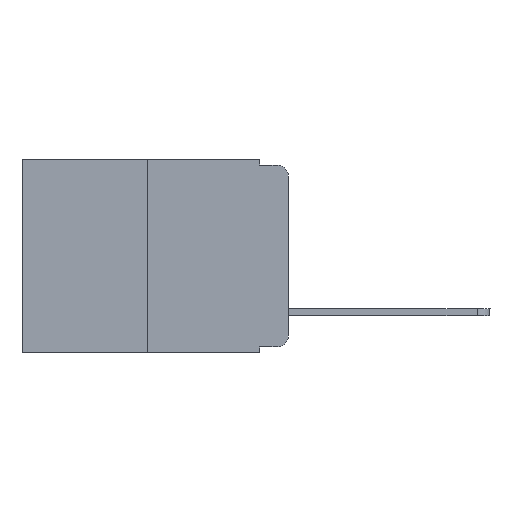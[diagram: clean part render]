
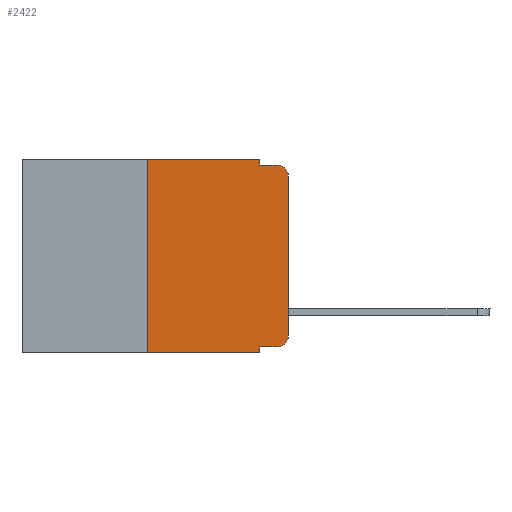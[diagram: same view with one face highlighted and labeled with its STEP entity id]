
A CAD part, left-side view. The second image highlights one B-rep face of the part: STEP entity #2422.
In plain terms, the highlighted planar face has unit normal (-1, 0, 0).
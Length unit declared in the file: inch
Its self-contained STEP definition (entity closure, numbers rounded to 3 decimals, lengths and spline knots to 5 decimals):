
#66 = CARTESIAN_POINT ( 'NONE',  ( 0., 0.25, 0. ) ) ;
#70 = CARTESIAN_POINT ( 'NONE',  ( 0., 0.051, -0.333 ) ) ;
#91 = CARTESIAN_POINT ( 'NONE',  ( 0., 0., -0.313 ) ) ;
#331 = ORIENTED_EDGE ( 'NONE', *, *, #2631, .T. ) ;
#383 = CARTESIAN_POINT ( 'NONE',  ( 0., 0.051, 0. ) ) ;
#431 = CARTESIAN_POINT ( 'NONE',  ( 0., 0.051, -0.343 ) ) ;
#577 = DIRECTION ( 'NONE',  ( 0., 0., -1. ) ) ;
#606 = EDGE_CURVE ( 'NONE', #12456, #6065, #13124, .T. ) ;
#678 = ORIENTED_EDGE ( 'NONE', *, *, #8364, .F. ) ;
#809 = PLANE ( 'NONE',  #10566 ) ;
#844 = CARTESIAN_POINT ( 'NONE',  ( 0., 0.051, -0.01 ) ) ;
#884 = CARTESIAN_POINT ( 'NONE',  ( 0., 0.02, -0.01 ) ) ;
#1283 = CARTESIAN_POINT ( 'NONE',  ( 0., 0., 0. ) ) ;
#1516 = LINE ( 'NONE', #11764, #2070 ) ;
#1545 = DIRECTION ( 'NONE',  ( 0., 0., 1. ) ) ;
#1553 = CARTESIAN_POINT ( 'NONE',  ( 0., 0.051, -0.01 ) ) ;
#1584 = EDGE_CURVE ( 'NONE', #11818, #4936, #2706, .T. ) ;
#1667 = DIRECTION ( 'NONE',  ( 0., 0., -1. ) ) ;
#1796 = DIRECTION ( 'NONE',  ( 1., 0., 0. ) ) ;
#1848 = CIRCLE ( 'NONE', #9337, 0.02 ) ;
#2070 = VECTOR ( 'NONE', #577, 39.37008 ) ;
#2153 = LINE ( 'NONE', #12272, #10392 ) ;
#2422 = ADVANCED_FACE ( 'NONE', ( #10788 ), #809, .F. ) ;
#2631 = EDGE_CURVE ( 'NONE', #3599, #6007, #12322, .T. ) ;
#2706 = LINE ( 'NONE', #844, #4121 ) ;
#3123 = VERTEX_POINT ( 'NONE', #431 ) ;
#3368 = ORIENTED_EDGE ( 'NONE', *, *, #606, .F. ) ;
#3408 = DIRECTION ( 'NONE',  ( 0., 0., -1. ) ) ;
#3510 = VERTEX_POINT ( 'NONE', #91 ) ;
#3599 = VERTEX_POINT ( 'NONE', #6467 ) ;
#3924 = EDGE_CURVE ( 'NONE', #3599, #3123, #12708, .T. ) ;
#4121 = VECTOR ( 'NONE', #10142, 39.37008 ) ;
#4555 = DIRECTION ( 'NONE',  ( 0., 0., -1. ) ) ;
#4722 = ORIENTED_EDGE ( 'NONE', *, *, #5256, .T. ) ;
#4901 = CARTESIAN_POINT ( 'NONE',  ( 0., 0.473, 0. ) ) ;
#4936 = VERTEX_POINT ( 'NONE', #884 ) ;
#5237 = DIRECTION ( 'NONE',  ( 0., -1., 0. ) ) ;
#5256 = EDGE_CURVE ( 'NONE', #6007, #3510, #1848, .T. ) ;
#5392 = EDGE_LOOP ( 'NONE', ( #12470, #13160, #11959, #7307, #3368, #678, #12584, #7066, #331, #4722 ) ) ;
#5424 = CARTESIAN_POINT ( 'NONE',  ( 0., 0.051, 0. ) ) ;
#5482 = VERTEX_POINT ( 'NONE', #6631 ) ;
#5528 = EDGE_CURVE ( 'NONE', #6065, #11818, #1516, .T. ) ;
#5584 = CARTESIAN_POINT ( 'NONE',  ( 0., 0.25, 0. ) ) ;
#5671 = EDGE_CURVE ( 'NONE', #3510, #5482, #6401, .T. ) ;
#5672 = EDGE_CURVE ( 'NONE', #8220, #3123, #2153, .T. ) ;
#6007 = VERTEX_POINT ( 'NONE', #6176 ) ;
#6065 = VERTEX_POINT ( 'NONE', #383 ) ;
#6118 = DIRECTION ( 'NONE',  ( 0., -1., 0. ) ) ;
#6159 = AXIS2_PLACEMENT_3D ( 'NONE', #7482, #10285, #12546 ) ;
#6176 = CARTESIAN_POINT ( 'NONE',  ( 0., 0.02, -0.333 ) ) ;
#6401 = LINE ( 'NONE', #1283, #6568 ) ;
#6467 = CARTESIAN_POINT ( 'NONE',  ( 0., 0.051, -0.333 ) ) ;
#6538 = EDGE_CURVE ( 'NONE', #5482, #4936, #7645, .T. ) ;
#6568 = VECTOR ( 'NONE', #10196, 39.37008 ) ;
#6631 = CARTESIAN_POINT ( 'NONE',  ( 0., 0., -0.03 ) ) ;
#6787 = LINE ( 'NONE', #5584, #8789 ) ;
#7066 = ORIENTED_EDGE ( 'NONE', *, *, #3924, .F. ) ;
#7307 = ORIENTED_EDGE ( 'NONE', *, *, #5528, .F. ) ;
#7482 = CARTESIAN_POINT ( 'NONE',  ( 0., 0.02, -0.03 ) ) ;
#7645 = CIRCLE ( 'NONE', #6159, 0.02 ) ;
#8220 = VERTEX_POINT ( 'NONE', #10468 ) ;
#8364 = EDGE_CURVE ( 'NONE', #8220, #12456, #6787, .T. ) ;
#8789 = VECTOR ( 'NONE', #1545, 39.37008 ) ;
#9337 = AXIS2_PLACEMENT_3D ( 'NONE', #10518, #12585, #3408 ) ;
#9461 = VECTOR ( 'NONE', #11072, 39.37008 ) ;
#10142 = DIRECTION ( 'NONE',  ( 0., -1., 0. ) ) ;
#10196 = DIRECTION ( 'NONE',  ( 0., 0., 1. ) ) ;
#10285 = DIRECTION ( 'NONE',  ( -1., 0., 0. ) ) ;
#10392 = VECTOR ( 'NONE', #5237, 39.37008 ) ;
#10468 = CARTESIAN_POINT ( 'NONE',  ( 0., 0.25, -0.343 ) ) ;
#10518 = CARTESIAN_POINT ( 'NONE',  ( 0., 0.02, -0.313 ) ) ;
#10566 = AXIS2_PLACEMENT_3D ( 'NONE', #11995, #1796, #1667 ) ;
#10787 = VECTOR ( 'NONE', #6118, 39.37008 ) ;
#10788 = FACE_OUTER_BOUND ( 'NONE', #5392, .T. ) ;
#11072 = DIRECTION ( 'NONE',  ( 0., -1., 0. ) ) ;
#11764 = CARTESIAN_POINT ( 'NONE',  ( 0., 0.051, 0. ) ) ;
#11818 = VERTEX_POINT ( 'NONE', #1553 ) ;
#11874 = VECTOR ( 'NONE', #4555, 39.37008 ) ;
#11959 = ORIENTED_EDGE ( 'NONE', *, *, #1584, .F. ) ;
#11995 = CARTESIAN_POINT ( 'NONE',  ( 0., 0.473, 0. ) ) ;
#12272 = CARTESIAN_POINT ( 'NONE',  ( 0., 0.473, -0.343 ) ) ;
#12322 = LINE ( 'NONE', #70, #10787 ) ;
#12456 = VERTEX_POINT ( 'NONE', #66 ) ;
#12470 = ORIENTED_EDGE ( 'NONE', *, *, #5671, .T. ) ;
#12546 = DIRECTION ( 'NONE',  ( 0., 0., -1. ) ) ;
#12584 = ORIENTED_EDGE ( 'NONE', *, *, #5672, .T. ) ;
#12585 = DIRECTION ( 'NONE',  ( -1., 0., 0. ) ) ;
#12708 = LINE ( 'NONE', #5424, #11874 ) ;
#13124 = LINE ( 'NONE', #4901, #9461 ) ;
#13160 = ORIENTED_EDGE ( 'NONE', *, *, #6538, .T. ) ;
